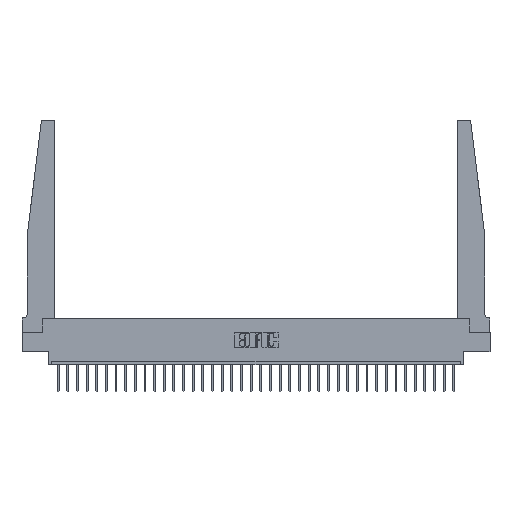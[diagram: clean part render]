
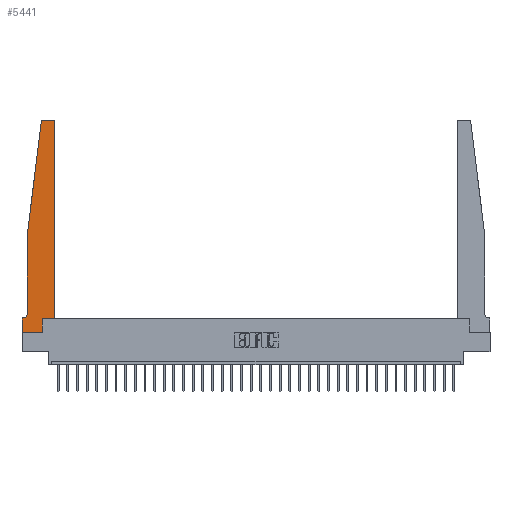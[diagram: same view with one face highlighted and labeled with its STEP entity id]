
A CAD part, top view. The second image highlights one B-rep face of the part: STEP entity #5441.
In plain terms, the highlighted planar face has unit normal (0, 0, 1).
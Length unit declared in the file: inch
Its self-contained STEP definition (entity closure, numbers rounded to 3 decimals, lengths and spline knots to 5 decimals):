
#33 = CARTESIAN_POINT ( 'NONE',  ( 0.065, 0.2375, 0.37 ) ) ;
#59 = VERTEX_POINT ( 'NONE', #20861 ) ;
#603 = ORIENTED_EDGE ( 'NONE', *, *, #11014, .T. ) ;
#1519 = DIRECTION ( 'NONE',  ( 0., 0., 1. ) ) ;
#1810 = AXIS2_PLACEMENT_3D ( 'NONE', #30187, #1519, #3956 ) ;
#1925 = VECTOR ( 'NONE', #21579, 39.37008 ) ;
#1954 = VECTOR ( 'NONE', #20632, 39.37008 ) ;
#1984 = VECTOR ( 'NONE', #4383, 39.37008 ) ;
#3315 = EDGE_CURVE ( 'NONE', #59, #30625, #28724, .T. ) ;
#3382 = DIRECTION ( 'NONE',  ( 0., 1., 0. ) ) ;
#3935 = DIRECTION ( 'NONE',  ( 1., 0., 0. ) ) ;
#3956 = DIRECTION ( 'NONE',  ( 1., 0., 0. ) ) ;
#4154 = ORIENTED_EDGE ( 'NONE', *, *, #24016, .T. ) ;
#4383 = DIRECTION ( 'NONE',  ( 0., -1., 0. ) ) ;
#4829 = LINE ( 'NONE', #12187, #29101 ) ;
#5441 = ADVANCED_FACE ( 'NONE', ( #21990 ), #25259, .T. ) ;
#5660 = DIRECTION ( 'NONE',  ( 0., 0., -1. ) ) ;
#6294 = CARTESIAN_POINT ( 'NONE',  ( 0.425, 2.72, 0.37 ) ) ;
#6928 = CARTESIAN_POINT ( 'NONE',  ( 0.425, 0.18, 0.37 ) ) ;
#7989 = LINE ( 'NONE', #8543, #1984 ) ;
#8060 = ORIENTED_EDGE ( 'NONE', *, *, #20050, .T. ) ;
#8282 = VECTOR ( 'NONE', #3382, 39.37008 ) ;
#8307 = VERTEX_POINT ( 'NONE', #23198 ) ;
#8543 = CARTESIAN_POINT ( 'NONE',  ( 0.065, 1.25, 0.37 ) ) ;
#8849 = ORIENTED_EDGE ( 'NONE', *, *, #3315, .T. ) ;
#9385 = CARTESIAN_POINT ( 'NONE',  ( 0.395, 2.72, 0.37 ) ) ;
#10488 = CARTESIAN_POINT ( 'NONE',  ( 0.2605, 0.18, 0.37 ) ) ;
#11014 = EDGE_CURVE ( 'NONE', #12962, #29013, #28901, .T. ) ;
#11236 = ORIENTED_EDGE ( 'NONE', *, *, #18947, .T. ) ;
#11493 = EDGE_CURVE ( 'NONE', #29013, #16190, #26998, .T. ) ;
#11519 = DIRECTION ( 'NONE',  ( 0., 0., 1. ) ) ;
#11659 = LINE ( 'NONE', #28587, #1925 ) ;
#12154 = ORIENTED_EDGE ( 'NONE', *, *, #18622, .T. ) ;
#12187 = CARTESIAN_POINT ( 'NONE',  ( 0., 0., 0.37 ) ) ;
#12962 = VERTEX_POINT ( 'NONE', #6294 ) ;
#13056 = DIRECTION ( 'NONE',  ( 0., -1., 0. ) ) ;
#13400 = CARTESIAN_POINT ( 'NONE',  ( 0.2605, 0.18, 0.37 ) ) ;
#13765 = AXIS2_PLACEMENT_3D ( 'NONE', #9385, #26103, #16180 ) ;
#14653 = CARTESIAN_POINT ( 'NONE',  ( 0.27653, 2.75, 0.37 ) ) ;
#14668 = EDGE_CURVE ( 'NONE', #14777, #59, #4829, .T. ) ;
#14777 = VERTEX_POINT ( 'NONE', #25773 ) ;
#14935 = VERTEX_POINT ( 'NONE', #33 ) ;
#15619 = ORIENTED_EDGE ( 'NONE', *, *, #18117, .T. ) ;
#15936 = ORIENTED_EDGE ( 'NONE', *, *, #30159, .T. ) ;
#16144 = CARTESIAN_POINT ( 'NONE',  ( 0.27653, 2.72, 0.37 ) ) ;
#16180 = DIRECTION ( 'NONE',  ( 1., 0., 0. ) ) ;
#16190 = VERTEX_POINT ( 'NONE', #14653 ) ;
#16444 = ORIENTED_EDGE ( 'NONE', *, *, #26164, .T. ) ;
#16682 = ORIENTED_EDGE ( 'NONE', *, *, #21169, .T. ) ;
#16963 = CARTESIAN_POINT ( 'NONE',  ( 0.065, 1.25, 0.37 ) ) ;
#17254 = LINE ( 'NONE', #10488, #8282 ) ;
#17703 = DIRECTION ( 'NONE',  ( 1., 0., 0. ) ) ;
#18014 = CARTESIAN_POINT ( 'NONE',  ( 0.25, 2.75, 0.37 ) ) ;
#18117 = EDGE_CURVE ( 'NONE', #16190, #30083, #23311, .T. ) ;
#18622 = EDGE_CURVE ( 'NONE', #8307, #14935, #7989, .T. ) ;
#18947 = EDGE_CURVE ( 'NONE', #30083, #8307, #24014, .T. ) ;
#18959 = VERTEX_POINT ( 'NONE', #25090 ) ;
#19547 = VECTOR ( 'NONE', #26041, 39.37008 ) ;
#19635 = ORIENTED_EDGE ( 'NONE', *, *, #11493, .T. ) ;
#20050 = EDGE_CURVE ( 'NONE', #30625, #23688, #17254, .T. ) ;
#20319 = LINE ( 'NONE', #6928, #19547 ) ;
#20632 = DIRECTION ( 'NONE',  ( -1., 0., 0. ) ) ;
#20861 = CARTESIAN_POINT ( 'NONE',  ( 0., 0., 0.37 ) ) ;
#20887 = LINE ( 'NONE', #25237, #22743 ) ;
#21041 = EDGE_LOOP ( 'NONE', ( #19635, #15619, #11236, #12154, #16682, #4154, #26198, #8849, #8060, #16444, #15936, #603 ) ) ;
#21169 = EDGE_CURVE ( 'NONE', #14935, #18959, #24605, .T. ) ;
#21298 = AXIS2_PLACEMENT_3D ( 'NONE', #16144, #11519, #30770 ) ;
#21579 = DIRECTION ( 'NONE',  ( -1., 0., 0. ) ) ;
#21990 = FACE_OUTER_BOUND ( 'NONE', #21041, .T. ) ;
#22743 = VECTOR ( 'NONE', #3935, 39.37008 ) ;
#23176 = CARTESIAN_POINT ( 'NONE',  ( 0.2605, 0., 0.37 ) ) ;
#23198 = CARTESIAN_POINT ( 'NONE',  ( 0.065, 1.25, 0.37 ) ) ;
#23224 = CARTESIAN_POINT ( 'NONE',  ( 0.425, 0.18, 0.37 ) ) ;
#23279 = VECTOR ( 'NONE', #29252, 39.37008 ) ;
#23311 = CIRCLE ( 'NONE', #21298, 0.03 ) ;
#23688 = VERTEX_POINT ( 'NONE', #13400 ) ;
#24014 = LINE ( 'NONE', #16963, #23279 ) ;
#24016 = EDGE_CURVE ( 'NONE', #18959, #14777, #11659, .T. ) ;
#24605 = CIRCLE ( 'NONE', #29227, 0.05 ) ;
#24971 = CARTESIAN_POINT ( 'NONE',  ( 0.015, 0.2375, 0.37 ) ) ;
#25090 = CARTESIAN_POINT ( 'NONE',  ( 0.015, 0.1875, 0.37 ) ) ;
#25237 = CARTESIAN_POINT ( 'NONE',  ( 0.425, 0.18, 0.37 ) ) ;
#25259 = PLANE ( 'NONE',  #1810 ) ;
#25773 = CARTESIAN_POINT ( 'NONE',  ( 0., 0.1875, 0.37 ) ) ;
#25934 = CARTESIAN_POINT ( 'NONE',  ( 0.24675, 2.72367, 0.37 ) ) ;
#26041 = DIRECTION ( 'NONE',  ( 0., 1., 0. ) ) ;
#26103 = DIRECTION ( 'NONE',  ( 0., 0., 1. ) ) ;
#26164 = EDGE_CURVE ( 'NONE', #23688, #29253, #20887, .T. ) ;
#26198 = ORIENTED_EDGE ( 'NONE', *, *, #14668, .T. ) ;
#26869 = VECTOR ( 'NONE', #17703, 39.37008 ) ;
#26944 = DIRECTION ( 'NONE',  ( -1., 0., 0. ) ) ;
#26998 = LINE ( 'NONE', #18014, #1954 ) ;
#28587 = CARTESIAN_POINT ( 'NONE',  ( 0.065, 0.1875, 0.37 ) ) ;
#28724 = LINE ( 'NONE', #29400, #26869 ) ;
#28901 = CIRCLE ( 'NONE', #13765, 0.03 ) ;
#28907 = CARTESIAN_POINT ( 'NONE',  ( 0.395, 2.75, 0.37 ) ) ;
#29013 = VERTEX_POINT ( 'NONE', #28907 ) ;
#29101 = VECTOR ( 'NONE', #13056, 39.37008 ) ;
#29227 = AXIS2_PLACEMENT_3D ( 'NONE', #24971, #5660, #26944 ) ;
#29252 = DIRECTION ( 'NONE',  ( -0.122, -0.992, 0. ) ) ;
#29253 = VERTEX_POINT ( 'NONE', #23224 ) ;
#29400 = CARTESIAN_POINT ( 'NONE',  ( 0., 0., 0.37 ) ) ;
#30083 = VERTEX_POINT ( 'NONE', #25934 ) ;
#30159 = EDGE_CURVE ( 'NONE', #29253, #12962, #20319, .T. ) ;
#30187 = CARTESIAN_POINT ( 'NONE',  ( 0., 0.1875, 0.37 ) ) ;
#30625 = VERTEX_POINT ( 'NONE', #23176 ) ;
#30770 = DIRECTION ( 'NONE',  ( 1., 0., 0. ) ) ;
